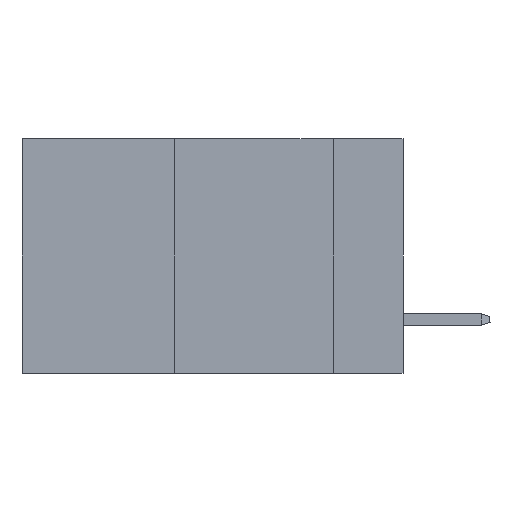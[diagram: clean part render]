
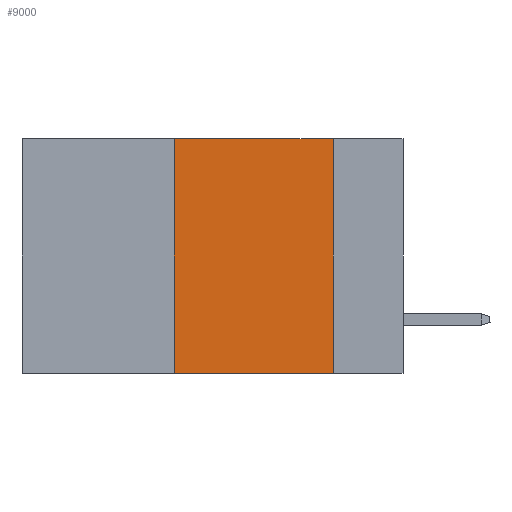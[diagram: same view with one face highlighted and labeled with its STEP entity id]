
A CAD part, left-side view. The second image highlights one B-rep face of the part: STEP entity #9000.
In plain terms, the highlighted planar face has unit normal (-1, 0, 0).
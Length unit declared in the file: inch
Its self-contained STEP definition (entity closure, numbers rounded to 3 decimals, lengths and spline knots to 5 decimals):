
#321 = ORIENTED_EDGE ( 'NONE', *, *, #5589, .T. ) ;
#688 = CARTESIAN_POINT ( 'NONE',  ( 0., 0.11, 0. ) ) ;
#1098 = VERTEX_POINT ( 'NONE', #19759 ) ;
#1232 = EDGE_CURVE ( 'NONE', #17890, #22727, #10260, .T. ) ;
#1458 = EDGE_CURVE ( 'NONE', #23205, #17890, #23021, .T. ) ;
#1464 = EDGE_LOOP ( 'NONE', ( #2637, #17021, #20897, #321 ) ) ;
#1504 = EDGE_CURVE ( 'NONE', #22727, #1098, #17455, .T. ) ;
#1537 = AXIS2_PLACEMENT_3D ( 'NONE', #3349, #13063, #16868 ) ;
#2637 = ORIENTED_EDGE ( 'NONE', *, *, #1504, .F. ) ;
#3349 = CARTESIAN_POINT ( 'NONE',  ( 0., 0.6, 0. ) ) ;
#3822 = VECTOR ( 'NONE', #24046, 39.37008 ) ;
#5414 = CARTESIAN_POINT ( 'NONE',  ( 0., 0.6, -0.37 ) ) ;
#5589 = EDGE_CURVE ( 'NONE', #23205, #1098, #22730, .T. ) ;
#5923 = CARTESIAN_POINT ( 'NONE',  ( 0., 0.36, 0. ) ) ;
#7014 = PLANE ( 'NONE',  #1537 ) ;
#8618 = CARTESIAN_POINT ( 'NONE',  ( 0., 0.6, 0. ) ) ;
#9000 = ADVANCED_FACE ( 'NONE', ( #13194 ), #7014, .F. ) ;
#10260 = LINE ( 'NONE', #8618, #3822 ) ;
#13063 = DIRECTION ( 'NONE',  ( 1., 0., 0. ) ) ;
#13194 = FACE_OUTER_BOUND ( 'NONE', #1464, .T. ) ;
#13401 = DIRECTION ( 'NONE',  ( 0., 0., 1. ) ) ;
#13901 = CARTESIAN_POINT ( 'NONE',  ( 0., 0.36, 0. ) ) ;
#16542 = DIRECTION ( 'NONE',  ( 0., -1., 0. ) ) ;
#16820 = VECTOR ( 'NONE', #16542, 39.37008 ) ;
#16868 = DIRECTION ( 'NONE',  ( 0., 0., -1. ) ) ;
#17021 = ORIENTED_EDGE ( 'NONE', *, *, #1232, .F. ) ;
#17455 = LINE ( 'NONE', #19100, #19154 ) ;
#17890 = VERTEX_POINT ( 'NONE', #5923 ) ;
#18609 = CARTESIAN_POINT ( 'NONE',  ( 0., 0.36, -0.37 ) ) ;
#19100 = CARTESIAN_POINT ( 'NONE',  ( 0., 0.11, 0. ) ) ;
#19154 = VECTOR ( 'NONE', #19230, 39.37008 ) ;
#19230 = DIRECTION ( 'NONE',  ( 0., 0., -1. ) ) ;
#19759 = CARTESIAN_POINT ( 'NONE',  ( 0., 0.11, -0.37 ) ) ;
#20897 = ORIENTED_EDGE ( 'NONE', *, *, #1458, .F. ) ;
#21978 = VECTOR ( 'NONE', #13401, 39.37008 ) ;
#22727 = VERTEX_POINT ( 'NONE', #688 ) ;
#22730 = LINE ( 'NONE', #5414, #16820 ) ;
#23021 = LINE ( 'NONE', #13901, #21978 ) ;
#23205 = VERTEX_POINT ( 'NONE', #18609 ) ;
#24046 = DIRECTION ( 'NONE',  ( 0., -1., 0. ) ) ;
